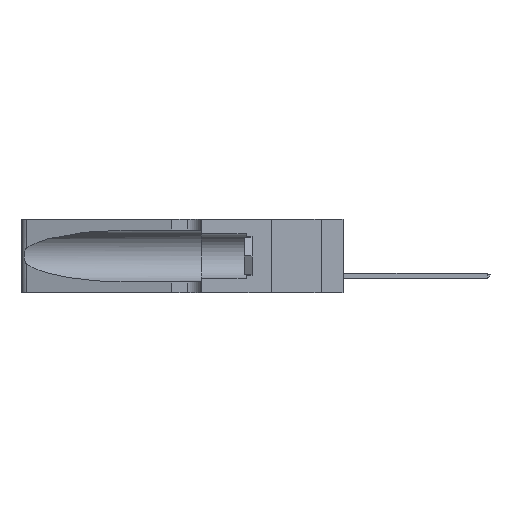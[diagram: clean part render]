
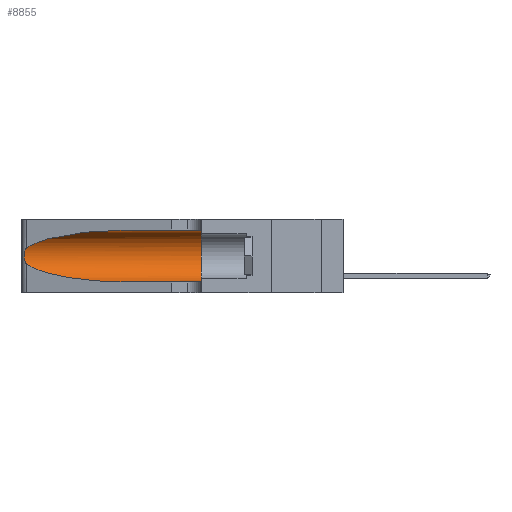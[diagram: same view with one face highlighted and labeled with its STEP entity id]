
A CAD part, left-side view. The second image highlights one B-rep face of the part: STEP entity #8855.
In plain terms, the highlighted cylindrical face has radius 3.308 mm (diameter 6.617 mm), a partial arc.
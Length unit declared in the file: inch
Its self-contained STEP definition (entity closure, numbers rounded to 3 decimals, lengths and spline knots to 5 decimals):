
#3 = CARTESIAN_POINT ( 'NONE',  ( 0.18966, 0.96281, 0.31525 ) ) ;
#229 = CARTESIAN_POINT ( 'NONE',  ( 0.1305, 0.72297, 0.31525 ) ) ;
#1453 = DIRECTION ( 'NONE',  ( 0., -1., 0. ) ) ;
#1869 =( BOUNDED_CURVE ( )  B_SPLINE_CURVE ( 3, ( #229, #3, #11636, #2719 ),
 .UNSPECIFIED., .F., .F. ) 
 B_SPLINE_CURVE_WITH_KNOTS ( ( 4, 4 ),
 ( 1.5708, 2.84003 ),
 .UNSPECIFIED. ) 
 CURVE ( )  GEOMETRIC_REPRESENTATION_ITEM ( )  RATIONAL_B_SPLINE_CURVE ( ( 1., 0.87, 0.87, 1. ) ) 
 REPRESENTATION_ITEM ( '' )  );
#2316 = DIRECTION ( 'NONE',  ( 0., -1., 0. ) ) ;
#2549 = CARTESIAN_POINT ( 'NONE',  ( 0.1305, 1.61858, 0.31525 ) ) ;
#2719 = CARTESIAN_POINT ( 'NONE',  ( 0.25487, 1.22718, 0.22369 ) ) ;
#2974 = VECTOR ( 'NONE', #1453, 39.37008 ) ;
#5058 = AXIS2_PLACEMENT_3D ( 'NONE', #14315, #20245, #34312 ) ;
#6101 = EDGE_CURVE ( 'NONE', #36272, #16227, #34997, .T. ) ;
#6915 = VERTEX_POINT ( 'NONE', #28834 ) ;
#7132 = EDGE_CURVE ( 'NONE', #12411, #16227, #35371, .T. ) ;
#7280 = CARTESIAN_POINT ( 'NONE',  ( 0.25787, 1.23484, 0.2124 ) ) ;
#7410 = CARTESIAN_POINT ( 'NONE',  ( 0.25487, 1.22718, 0.22369 ) ) ;
#7756 = VECTOR ( 'NONE', #2316, 39.37008 ) ;
#7793 = CARTESIAN_POINT ( 'NONE',  ( 0.26018, 1.23835, 0.19895 ) ) ;
#8855 = ADVANCED_FACE ( 'NONE', ( #33580 ), #19347, .F. ) ;
#10162 = CARTESIAN_POINT ( 'NONE',  ( 0.25854, 1.2359, 0.20912 ) ) ;
#11109 = EDGE_CURVE ( 'NONE', #15564, #16352, #11204, .T. ) ;
#11161 = CARTESIAN_POINT ( 'NONE',  ( 0.25487, 1.22718, 0.14631 ) ) ;
#11196 = CARTESIAN_POINT ( 'NONE',  ( 0.25487, 1.22718, 0.14631 ) ) ;
#11204 = B_SPLINE_CURVE_WITH_KNOTS ( 'NONE', 3,
 ( #7410, #29677, #32645, #7280, #10162, #7793, #33398, #27946, #27440, #19230, #22063, #19103, #20043, #11161 ),
 .UNSPECIFIED., .F., .F.,
 ( 4, 2, 2, 2, 2, 2, 4 ),
 ( 0., 0.00027, 0.00053, 0.00107, 0.0016, 0.00187, 0.00214 ),
 .UNSPECIFIED. ) ;
#11636 = CARTESIAN_POINT ( 'NONE',  ( 0.2373, 1.15595, 0.28018 ) ) ;
#12411 = VERTEX_POINT ( 'NONE', #20820 ) ;
#14315 = CARTESIAN_POINT ( 'NONE',  ( 0.1305, 1.61858, 0.185 ) ) ;
#14665 = ORIENTED_EDGE ( 'NONE', *, *, #11109, .T. ) ;
#15564 = VERTEX_POINT ( 'NONE', #35283 ) ;
#15862 = CARTESIAN_POINT ( 'NONE',  ( 0.1305, 1.61858, 0.05475 ) ) ;
#16204 =( BOUNDED_CURVE ( )  B_SPLINE_CURVE ( 3, ( #11196, #23215, #19634, #19517 ),
 .UNSPECIFIED., .F., .F. ) 
 B_SPLINE_CURVE_WITH_KNOTS ( ( 4, 4 ),
 ( 3.44316, 4.71239 ),
 .UNSPECIFIED. ) 
 CURVE ( )  GEOMETRIC_REPRESENTATION_ITEM ( )  RATIONAL_B_SPLINE_CURVE ( ( 1., 0.87, 0.87, 1. ) ) 
 REPRESENTATION_ITEM ( '' )  );
#16227 = VERTEX_POINT ( 'NONE', #22599 ) ;
#16352 = VERTEX_POINT ( 'NONE', #21571 ) ;
#16541 = ORIENTED_EDGE ( 'NONE', *, *, #33250, .T. ) ;
#19103 = CARTESIAN_POINT ( 'NONE',  ( 0.25639, 1.23186, 0.15144 ) ) ;
#19230 = CARTESIAN_POINT ( 'NONE',  ( 0.25856, 1.23593, 0.16098 ) ) ;
#19347 = CYLINDRICAL_SURFACE ( 'NONE', #5058, 0.13025 ) ;
#19517 = CARTESIAN_POINT ( 'NONE',  ( 0.1305, 0.72297, 0.05475 ) ) ;
#19634 = CARTESIAN_POINT ( 'NONE',  ( 0.18966, 0.96281, 0.05475 ) ) ;
#20043 = CARTESIAN_POINT ( 'NONE',  ( 0.25555, 1.22993, 0.14849 ) ) ;
#20245 = DIRECTION ( 'NONE',  ( 0., -1., 0. ) ) ;
#20820 = CARTESIAN_POINT ( 'NONE',  ( 0.1305, 0.35, 0.31525 ) ) ;
#20972 = DIRECTION ( 'NONE',  ( 0., 1., 0. ) ) ;
#21571 = CARTESIAN_POINT ( 'NONE',  ( 0.25487, 1.22718, 0.14631 ) ) ;
#22063 = CARTESIAN_POINT ( 'NONE',  ( 0.25789, 1.23486, 0.15765 ) ) ;
#22599 = CARTESIAN_POINT ( 'NONE',  ( 0.1305, 0.35, 0.05475 ) ) ;
#23215 = CARTESIAN_POINT ( 'NONE',  ( 0.2373, 1.15595, 0.08982 ) ) ;
#23849 = DIRECTION ( 'NONE',  ( 0., 0., 1. ) ) ;
#24463 = ORIENTED_EDGE ( 'NONE', *, *, #30200, .T. ) ;
#25679 = ORIENTED_EDGE ( 'NONE', *, *, #7132, .F. ) ;
#25912 = AXIS2_PLACEMENT_3D ( 'NONE', #35163, #20972, #23849 ) ;
#27064 = EDGE_LOOP ( 'NONE', ( #24463, #14665, #16541, #29560, #25679, #27327 ) ) ;
#27327 = ORIENTED_EDGE ( 'NONE', *, *, #32696, .F. ) ;
#27440 = CARTESIAN_POINT ( 'NONE',  ( 0.26017, 1.23833, 0.17102 ) ) ;
#27946 = CARTESIAN_POINT ( 'NONE',  ( 0.26075, 1.23896, 0.178 ) ) ;
#28834 = CARTESIAN_POINT ( 'NONE',  ( 0.1305, 0.72297, 0.31525 ) ) ;
#29534 = LINE ( 'NONE', #2549, #7756 ) ;
#29560 = ORIENTED_EDGE ( 'NONE', *, *, #6101, .T. ) ;
#29677 = CARTESIAN_POINT ( 'NONE',  ( 0.25555, 1.22994, 0.2215 ) ) ;
#30200 = EDGE_CURVE ( 'NONE', #6915, #15564, #1869, .T. ) ;
#32645 = CARTESIAN_POINT ( 'NONE',  ( 0.25639, 1.23184, 0.21858 ) ) ;
#32696 = EDGE_CURVE ( 'NONE', #6915, #12411, #29534, .T. ) ;
#33250 = EDGE_CURVE ( 'NONE', #16352, #36272, #16204, .T. ) ;
#33398 = CARTESIAN_POINT ( 'NONE',  ( 0.26075, 1.23896, 0.19203 ) ) ;
#33442 = CARTESIAN_POINT ( 'NONE',  ( 0.1305, 0.72297, 0.05475 ) ) ;
#33580 = FACE_OUTER_BOUND ( 'NONE', #27064, .T. ) ;
#34312 = DIRECTION ( 'NONE',  ( 0., 0., -1. ) ) ;
#34997 = LINE ( 'NONE', #15862, #2974 ) ;
#35163 = CARTESIAN_POINT ( 'NONE',  ( 0.1305, 0.35, 0.185 ) ) ;
#35283 = CARTESIAN_POINT ( 'NONE',  ( 0.25487, 1.22718, 0.22369 ) ) ;
#35371 = CIRCLE ( 'NONE', #25912, 0.13025 ) ;
#36272 = VERTEX_POINT ( 'NONE', #33442 ) ;
